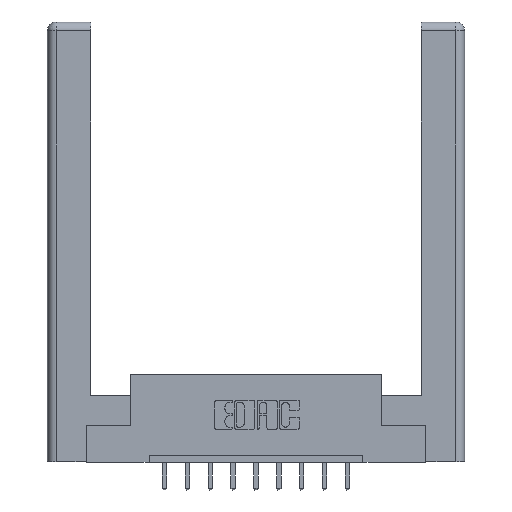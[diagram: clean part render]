
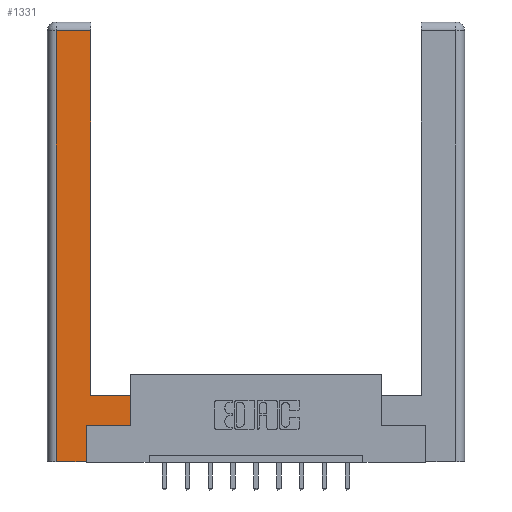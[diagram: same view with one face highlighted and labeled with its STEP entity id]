
A CAD part, top view. The second image highlights one B-rep face of the part: STEP entity #1331.
In plain terms, the highlighted planar face has unit normal (0, 0, 1).
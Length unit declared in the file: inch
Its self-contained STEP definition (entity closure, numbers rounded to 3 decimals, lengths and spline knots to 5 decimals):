
#173 = VERTEX_POINT ( 'NONE', #10692 ) ;
#186 = VERTEX_POINT ( 'NONE', #2181 ) ;
#365 = VERTEX_POINT ( 'NONE', #9286 ) ;
#568 = EDGE_CURVE ( 'NONE', #4802, #173, #12866, .T. ) ;
#575 = AXIS2_PLACEMENT_3D ( 'NONE', #13263, #6834, #3596 ) ;
#723 = DIRECTION ( 'NONE',  ( 0., -1., 0. ) ) ;
#1118 = LINE ( 'NONE', #10577, #8420 ) ;
#1331 = ADVANCED_FACE ( 'NONE', ( #11016 ), #12197, .F. ) ;
#1783 = VERTEX_POINT ( 'NONE', #10302 ) ;
#2181 = CARTESIAN_POINT ( 'NONE',  ( 0.265, 0., 0. ) ) ;
#2506 = ORIENTED_EDGE ( 'NONE', *, *, #11671, .T. ) ;
#2891 = CARTESIAN_POINT ( 'NONE',  ( 0.0615, 0., 0. ) ) ;
#2908 = CARTESIAN_POINT ( 'NONE',  ( 0.295, 0.45, 0. ) ) ;
#3171 = ORIENTED_EDGE ( 'NONE', *, *, #10436, .T. ) ;
#3220 = ORIENTED_EDGE ( 'NONE', *, *, #13411, .T. ) ;
#3258 = LINE ( 'NONE', #2908, #4586 ) ;
#3481 = LINE ( 'NONE', #2891, #12409 ) ;
#3596 = DIRECTION ( 'NONE',  ( -1., 0., 0. ) ) ;
#3783 = VECTOR ( 'NONE', #9683, 39.37008 ) ;
#4586 = VECTOR ( 'NONE', #9183, 39.37008 ) ;
#4754 = EDGE_CURVE ( 'NONE', #186, #4802, #9278, .T. ) ;
#4802 = VERTEX_POINT ( 'NONE', #10898 ) ;
#4949 = EDGE_CURVE ( 'NONE', #1783, #12469, #12420, .T. ) ;
#5113 = ORIENTED_EDGE ( 'NONE', *, *, #4949, .T. ) ;
#5394 = EDGE_CURVE ( 'NONE', #12208, #365, #3481, .T. ) ;
#5618 = DIRECTION ( 'NONE',  ( 0., 1., 0. ) ) ;
#5694 = DIRECTION ( 'NONE',  ( 0., 1., 0. ) ) ;
#5856 = DIRECTION ( 'NONE',  ( 0., 1., 0. ) ) ;
#5956 = VECTOR ( 'NONE', #5618, 39.37008 ) ;
#6228 = CARTESIAN_POINT ( 'NONE',  ( 0.295, 2.94, 0. ) ) ;
#6422 = LINE ( 'NONE', #11007, #5956 ) ;
#6460 = VECTOR ( 'NONE', #5694, 39.37008 ) ;
#6471 = VECTOR ( 'NONE', #5856, 39.37008 ) ;
#6804 = CARTESIAN_POINT ( 'NONE',  ( 0.265, 0., 0. ) ) ;
#6820 = CARTESIAN_POINT ( 'NONE',  ( 0.265, 0.245, 0. ) ) ;
#6834 = DIRECTION ( 'NONE',  ( 0., 0., -1. ) ) ;
#7283 = VECTOR ( 'NONE', #12300, 39.37008 ) ;
#7443 = ORIENTED_EDGE ( 'NONE', *, *, #568, .T. ) ;
#7890 = CARTESIAN_POINT ( 'NONE',  ( 0.0615, 2.94, 0. ) ) ;
#8123 = LINE ( 'NONE', #6804, #7283 ) ;
#8420 = VECTOR ( 'NONE', #11745, 39.37008 ) ;
#8773 = CARTESIAN_POINT ( 'NONE',  ( 0.565, 0.245, 0. ) ) ;
#8925 = EDGE_CURVE ( 'NONE', #365, #186, #8123, .T. ) ;
#9183 = DIRECTION ( 'NONE',  ( -1., 0., 0. ) ) ;
#9278 = LINE ( 'NONE', #6820, #6471 ) ;
#9286 = CARTESIAN_POINT ( 'NONE',  ( 0.0615, 0., 0. ) ) ;
#9374 = CARTESIAN_POINT ( 'NONE',  ( 0.565, 0.45, 0. ) ) ;
#9683 = DIRECTION ( 'NONE',  ( 1., 0., 0. ) ) ;
#10302 = CARTESIAN_POINT ( 'NONE',  ( 0.295, 0.45, 0. ) ) ;
#10436 = EDGE_CURVE ( 'NONE', #12469, #12208, #1118, .T. ) ;
#10577 = CARTESIAN_POINT ( 'NONE',  ( 0.0615, 2.94, 0. ) ) ;
#10692 = CARTESIAN_POINT ( 'NONE',  ( 0.565, 0.245, 0. ) ) ;
#10720 = EDGE_LOOP ( 'NONE', ( #5113, #3171, #13636, #12780, #13395, #7443, #3220, #2506 ) ) ;
#10898 = CARTESIAN_POINT ( 'NONE',  ( 0.265, 0.245, 0. ) ) ;
#11007 = CARTESIAN_POINT ( 'NONE',  ( 0.565, 0.45, 0. ) ) ;
#11016 = FACE_OUTER_BOUND ( 'NONE', #10720, .T. ) ;
#11129 = CARTESIAN_POINT ( 'NONE',  ( 0.295, 3., 0. ) ) ;
#11671 = EDGE_CURVE ( 'NONE', #13715, #1783, #3258, .T. ) ;
#11745 = DIRECTION ( 'NONE',  ( -1., 0., 0. ) ) ;
#12197 = PLANE ( 'NONE',  #575 ) ;
#12208 = VERTEX_POINT ( 'NONE', #7890 ) ;
#12300 = DIRECTION ( 'NONE',  ( 1., 0., 0. ) ) ;
#12409 = VECTOR ( 'NONE', #723, 39.37008 ) ;
#12420 = LINE ( 'NONE', #11129, #6460 ) ;
#12469 = VERTEX_POINT ( 'NONE', #6228 ) ;
#12780 = ORIENTED_EDGE ( 'NONE', *, *, #8925, .T. ) ;
#12866 = LINE ( 'NONE', #8773, #3783 ) ;
#13263 = CARTESIAN_POINT ( 'NONE',  ( 0., 0., 0. ) ) ;
#13395 = ORIENTED_EDGE ( 'NONE', *, *, #4754, .T. ) ;
#13411 = EDGE_CURVE ( 'NONE', #173, #13715, #6422, .T. ) ;
#13636 = ORIENTED_EDGE ( 'NONE', *, *, #5394, .T. ) ;
#13715 = VERTEX_POINT ( 'NONE', #9374 ) ;
